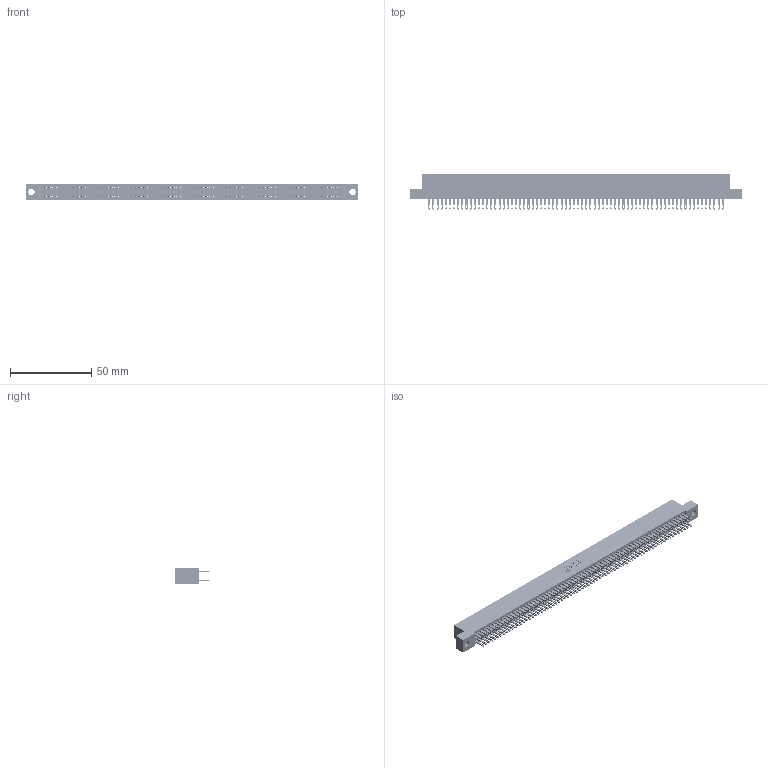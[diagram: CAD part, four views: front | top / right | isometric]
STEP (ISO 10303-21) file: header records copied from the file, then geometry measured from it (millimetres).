
FILE_DESCRIPTION (( 'STEP AP203' ), '1' );
FILE_NAME ('345-144-500-204.STEP', '2021-05-26T02:30:32', ( '' ), ( '' ), 'SwSTEP 2.0', 'SolidWorks 2020', '' );
FILE_SCHEMA (( 'CONFIG_CONTROL_DESIGN' ));
Length unit declared in the file: inch
Products named in the file (3): 345-144-500-204; 345 Part_Flush Mounting Lugs - 0.156 Dia-TI; 345-292-001_345-293-100
Assembly tree (145 placements, depth 2):
  345-144-500-204
    345 Part_Flush Mounting Lugs - 0.156 Dia-TI
    345-292-001_345-293-100  x144
Bounding box: 204.09 x 21.51 x 9.4 mm (x, y, z)
Volume: 20438 mm3; surface area: 32112.1 mm2
Topology: 145 solids, 145 shells, 6764 faces, 20681 edges, 13786 vertices
Faces by surface type: plane 3982, cylinder 2782
Entity records: 52803 total; most frequent: CARTESIAN_POINT 8826, ORIENTED_EDGE 8758, DIRECTION 7747, EDGE_CURVE 4379, VECTOR 3955, LINE 3955, VERTEX_POINT 2918, AXIS2_PLACEMENT_3D 1896
